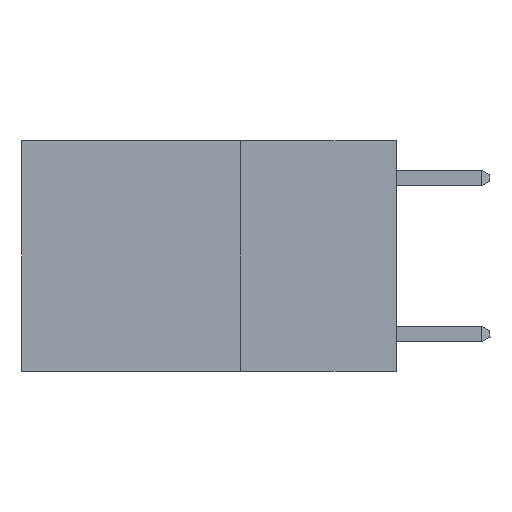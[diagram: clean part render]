
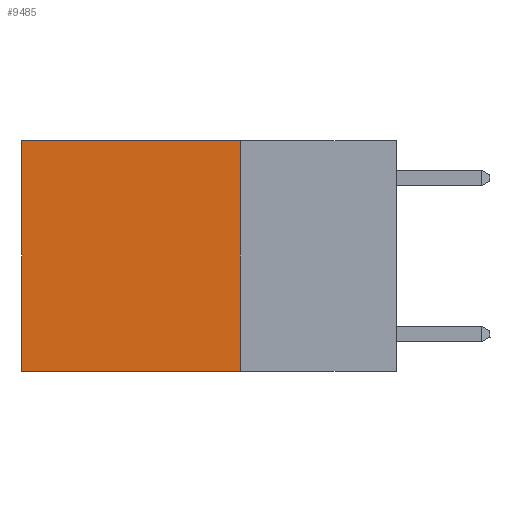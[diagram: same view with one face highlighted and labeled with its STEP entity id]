
A CAD part, left-side view. The second image highlights one B-rep face of the part: STEP entity #9485.
In plain terms, the highlighted planar face has unit normal (-1, 0, 0).
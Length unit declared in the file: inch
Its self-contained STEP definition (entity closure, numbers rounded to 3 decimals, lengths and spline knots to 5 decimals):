
#55 = VECTOR ( 'NONE', #4135, 39.37008 ) ;
#560 = ORIENTED_EDGE ( 'NONE', *, *, #7814, .F. ) ;
#927 = EDGE_CURVE ( 'NONE', #8774, #7118, #10211, .T. ) ;
#999 = VERTEX_POINT ( 'NONE', #4647 ) ;
#1091 = EDGE_CURVE ( 'NONE', #999, #8774, #4183, .T. ) ;
#2451 = VECTOR ( 'NONE', #5119, 39.37008 ) ;
#2676 = CARTESIAN_POINT ( 'NONE',  ( 0.2625, 0.6, -0.37 ) ) ;
#3014 = ORIENTED_EDGE ( 'NONE', *, *, #1091, .T. ) ;
#3261 = CARTESIAN_POINT ( 'NONE',  ( 0.2625, 0.25, -0.37 ) ) ;
#3939 = LINE ( 'NONE', #7835, #10081 ) ;
#4135 = DIRECTION ( 'NONE',  ( 0., 1., 0. ) ) ;
#4183 = LINE ( 'NONE', #7441, #55 ) ;
#4568 = DIRECTION ( 'NONE',  ( 0., 0., -1. ) ) ;
#4647 = CARTESIAN_POINT ( 'NONE',  ( 0.2625, 0.25, 0. ) ) ;
#4796 = EDGE_CURVE ( 'NONE', #999, #8971, #3939, .T. ) ;
#5119 = DIRECTION ( 'NONE',  ( 0., 1., 0. ) ) ;
#6172 = AXIS2_PLACEMENT_3D ( 'NONE', #10078, #9344, #4568 ) ;
#6283 = CARTESIAN_POINT ( 'NONE',  ( 0.2625, 0.6, 0. ) ) ;
#6372 = DIRECTION ( 'NONE',  ( 0., 0., -1. ) ) ;
#6678 = CARTESIAN_POINT ( 'NONE',  ( 0.2625, 0.25, -0.37 ) ) ;
#6773 = LINE ( 'NONE', #6678, #2451 ) ;
#6996 = EDGE_LOOP ( 'NONE', ( #8940, #560, #9192, #3014 ) ) ;
#7118 = VERTEX_POINT ( 'NONE', #2676 ) ;
#7441 = CARTESIAN_POINT ( 'NONE',  ( 0.2625, 0.25, 0. ) ) ;
#7814 = EDGE_CURVE ( 'NONE', #8971, #7118, #6773, .T. ) ;
#7835 = CARTESIAN_POINT ( 'NONE',  ( 0.2625, 0.25, 0. ) ) ;
#8535 = PLANE ( 'NONE',  #6172 ) ;
#8572 = VECTOR ( 'NONE', #6372, 39.37008 ) ;
#8647 = DIRECTION ( 'NONE',  ( 0., 0., -1. ) ) ;
#8774 = VERTEX_POINT ( 'NONE', #6283 ) ;
#8940 = ORIENTED_EDGE ( 'NONE', *, *, #927, .T. ) ;
#8971 = VERTEX_POINT ( 'NONE', #3261 ) ;
#9179 = FACE_OUTER_BOUND ( 'NONE', #6996, .T. ) ;
#9192 = ORIENTED_EDGE ( 'NONE', *, *, #4796, .F. ) ;
#9344 = DIRECTION ( 'NONE',  ( 1., 0., 0. ) ) ;
#9485 = ADVANCED_FACE ( 'NONE', ( #9179 ), #8535, .F. ) ;
#10078 = CARTESIAN_POINT ( 'NONE',  ( 0.2625, 0.25, 0. ) ) ;
#10081 = VECTOR ( 'NONE', #8647, 39.37008 ) ;
#10211 = LINE ( 'NONE', #10221, #8572 ) ;
#10221 = CARTESIAN_POINT ( 'NONE',  ( 0.2625, 0.6, 0. ) ) ;
